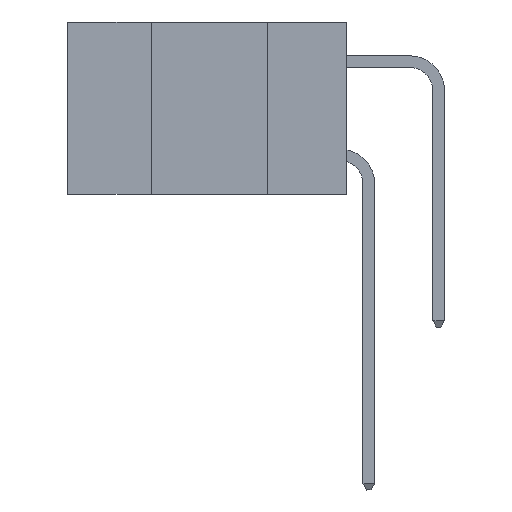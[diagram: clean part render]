
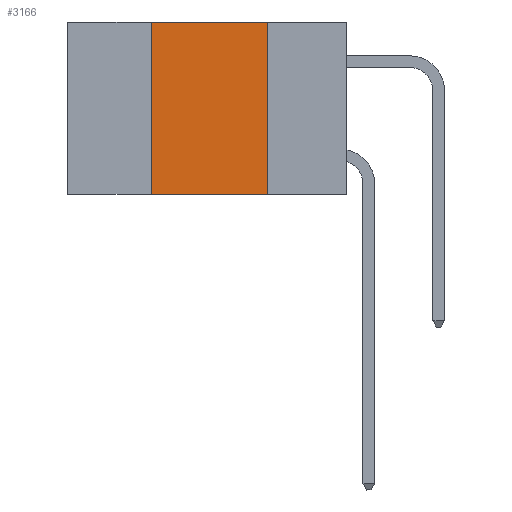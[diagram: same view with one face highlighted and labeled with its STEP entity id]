
A CAD part, left-side view. The second image highlights one B-rep face of the part: STEP entity #3166.
In plain terms, the highlighted planar face has unit normal (-1, 0, 0).
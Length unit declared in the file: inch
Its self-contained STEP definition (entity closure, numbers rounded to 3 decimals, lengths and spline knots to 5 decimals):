
#135 = CARTESIAN_POINT ( 'NONE',  ( 0., 0.42, 0. ) ) ;
#258 = LINE ( 'NONE', #135, #9477 ) ;
#709 = VERTEX_POINT ( 'NONE', #4847 ) ;
#712 = VECTOR ( 'NONE', #1208, 39.37008 ) ;
#793 = LINE ( 'NONE', #11640, #7921 ) ;
#824 = ORIENTED_EDGE ( 'NONE', *, *, #8397, .T. ) ;
#1064 = DIRECTION ( 'NONE',  ( 0., 0., -1. ) ) ;
#1208 = DIRECTION ( 'NONE',  ( 0., -1., 0. ) ) ;
#1375 = LINE ( 'NONE', #4775, #712 ) ;
#2761 = CARTESIAN_POINT ( 'NONE',  ( 0., 0.42, 0. ) ) ;
#3166 = ADVANCED_FACE ( 'NONE', ( #5695 ), #9275, .F. ) ;
#4312 = ORIENTED_EDGE ( 'NONE', *, *, #5205, .F. ) ;
#4693 = CARTESIAN_POINT ( 'NONE',  ( 0., 0.6, 0. ) ) ;
#4775 = CARTESIAN_POINT ( 'NONE',  ( 0., 0.6, -0.37 ) ) ;
#4847 = CARTESIAN_POINT ( 'NONE',  ( 0., 0.42, -0.37 ) ) ;
#5205 = EDGE_CURVE ( 'NONE', #6041, #10389, #8125, .T. ) ;
#5695 = FACE_OUTER_BOUND ( 'NONE', #10488, .T. ) ;
#6041 = VERTEX_POINT ( 'NONE', #2761 ) ;
#6077 = VERTEX_POINT ( 'NONE', #10017 ) ;
#6347 = DIRECTION ( 'NONE',  ( 0., -1., 0. ) ) ;
#6464 = CARTESIAN_POINT ( 'NONE',  ( 0., 0.6, 0. ) ) ;
#7921 = VECTOR ( 'NONE', #11460, 39.37008 ) ;
#8085 = AXIS2_PLACEMENT_3D ( 'NONE', #4693, #10175, #1064 ) ;
#8088 = EDGE_CURVE ( 'NONE', #10389, #6077, #793, .T. ) ;
#8125 = LINE ( 'NONE', #6464, #8394 ) ;
#8394 = VECTOR ( 'NONE', #6347, 39.37008 ) ;
#8397 = EDGE_CURVE ( 'NONE', #709, #6077, #1375, .T. ) ;
#8811 = ORIENTED_EDGE ( 'NONE', *, *, #8088, .F. ) ;
#9275 = PLANE ( 'NONE',  #8085 ) ;
#9364 = DIRECTION ( 'NONE',  ( 0., 0., 1. ) ) ;
#9477 = VECTOR ( 'NONE', #9364, 39.37008 ) ;
#10017 = CARTESIAN_POINT ( 'NONE',  ( 0., 0.17, -0.37 ) ) ;
#10175 = DIRECTION ( 'NONE',  ( 1., 0., 0. ) ) ;
#10389 = VERTEX_POINT ( 'NONE', #11006 ) ;
#10488 = EDGE_LOOP ( 'NONE', ( #8811, #4312, #11138, #824 ) ) ;
#11006 = CARTESIAN_POINT ( 'NONE',  ( 0., 0.17, 0. ) ) ;
#11138 = ORIENTED_EDGE ( 'NONE', *, *, #11290, .F. ) ;
#11290 = EDGE_CURVE ( 'NONE', #709, #6041, #258, .T. ) ;
#11460 = DIRECTION ( 'NONE',  ( 0., 0., -1. ) ) ;
#11640 = CARTESIAN_POINT ( 'NONE',  ( 0., 0.17, 0. ) ) ;
